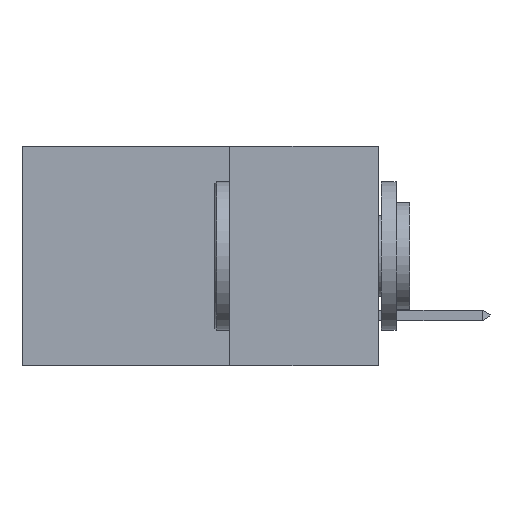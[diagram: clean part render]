
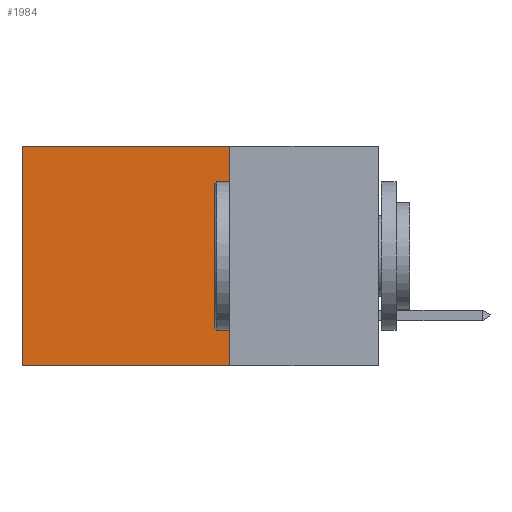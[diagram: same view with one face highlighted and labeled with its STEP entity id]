
A CAD part, left-side view. The second image highlights one B-rep face of the part: STEP entity #1984.
In plain terms, the highlighted planar face has unit normal (-1, 0, 0).
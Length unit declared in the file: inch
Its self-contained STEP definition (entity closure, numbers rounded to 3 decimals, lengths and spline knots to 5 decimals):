
#6 = CARTESIAN_POINT ( 'NONE',  ( 0.298, 0.25, -0.37 ) ) ;
#133 = DIRECTION ( 'NONE',  ( 0., 1., 0. ) ) ;
#1984 = ADVANCED_FACE ( 'NONE', ( #7303 ), #11754, .F. ) ;
#2307 = LINE ( 'NONE', #7315, #6517 ) ;
#2466 = VECTOR ( 'NONE', #9750, 39.37008 ) ;
#2512 = EDGE_CURVE ( 'NONE', #4511, #9515, #3665, .T. ) ;
#2825 = ORIENTED_EDGE ( 'NONE', *, *, #10738, .T. ) ;
#3196 = CARTESIAN_POINT ( 'NONE',  ( 0.298, 0.6, 0. ) ) ;
#3665 = LINE ( 'NONE', #10838, #2466 ) ;
#4000 = LINE ( 'NONE', #3196, #11179 ) ;
#4156 = DIRECTION ( 'NONE',  ( 0., 0., -1. ) ) ;
#4511 = VERTEX_POINT ( 'NONE', #7899 ) ;
#5877 = VERTEX_POINT ( 'NONE', #8197 ) ;
#6110 = CARTESIAN_POINT ( 'NONE',  ( 0.298, 0.25, 0. ) ) ;
#6185 = EDGE_LOOP ( 'NONE', ( #9579, #10213, #10633, #2825 ) ) ;
#6517 = VECTOR ( 'NONE', #10080, 39.37008 ) ;
#6980 = DIRECTION ( 'NONE',  ( 0., 0., -1. ) ) ;
#7303 = FACE_OUTER_BOUND ( 'NONE', #6185, .T. ) ;
#7315 = CARTESIAN_POINT ( 'NONE',  ( 0.298, 0.25, -0.37 ) ) ;
#7651 = VECTOR ( 'NONE', #133, 39.37008 ) ;
#7899 = CARTESIAN_POINT ( 'NONE',  ( 0.298, 0.25, 0. ) ) ;
#8055 = EDGE_CURVE ( 'NONE', #9515, #9231, #2307, .T. ) ;
#8197 = CARTESIAN_POINT ( 'NONE',  ( 0.298, 0.6, 0. ) ) ;
#8746 = CARTESIAN_POINT ( 'NONE',  ( 0.298, 0.25, 0. ) ) ;
#8921 = AXIS2_PLACEMENT_3D ( 'NONE', #6110, #9970, #6980 ) ;
#8970 = LINE ( 'NONE', #8746, #7651 ) ;
#9231 = VERTEX_POINT ( 'NONE', #10008 ) ;
#9515 = VERTEX_POINT ( 'NONE', #6 ) ;
#9579 = ORIENTED_EDGE ( 'NONE', *, *, #10918, .T. ) ;
#9750 = DIRECTION ( 'NONE',  ( 0., 0., -1. ) ) ;
#9970 = DIRECTION ( 'NONE',  ( 1., 0., 0. ) ) ;
#10008 = CARTESIAN_POINT ( 'NONE',  ( 0.298, 0.6, -0.37 ) ) ;
#10080 = DIRECTION ( 'NONE',  ( 0., 1., 0. ) ) ;
#10213 = ORIENTED_EDGE ( 'NONE', *, *, #8055, .F. ) ;
#10633 = ORIENTED_EDGE ( 'NONE', *, *, #2512, .F. ) ;
#10738 = EDGE_CURVE ( 'NONE', #4511, #5877, #8970, .T. ) ;
#10838 = CARTESIAN_POINT ( 'NONE',  ( 0.298, 0.25, 0. ) ) ;
#10918 = EDGE_CURVE ( 'NONE', #5877, #9231, #4000, .T. ) ;
#11179 = VECTOR ( 'NONE', #4156, 39.37008 ) ;
#11754 = PLANE ( 'NONE',  #8921 ) ;
